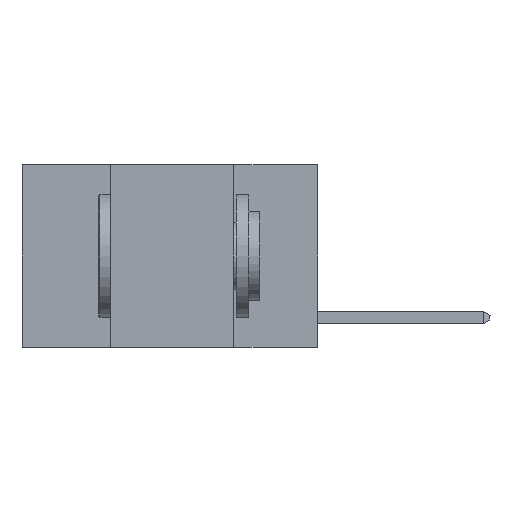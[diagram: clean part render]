
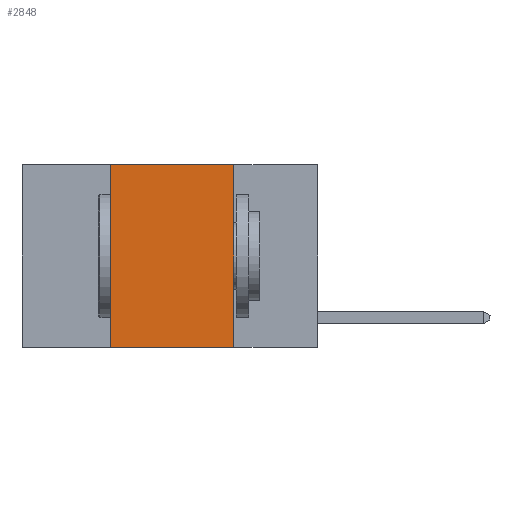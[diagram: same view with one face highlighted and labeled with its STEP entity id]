
A CAD part, left-side view. The second image highlights one B-rep face of the part: STEP entity #2848.
In plain terms, the highlighted planar face has unit normal (-1, 0, 0).
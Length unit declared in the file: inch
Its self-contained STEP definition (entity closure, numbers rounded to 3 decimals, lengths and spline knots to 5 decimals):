
#1011 = CARTESIAN_POINT ( 'NONE',  ( 0., 0.6, -0.37 ) ) ;
#1849 = ORIENTED_EDGE ( 'NONE', *, *, #4681, .T. ) ;
#1948 = LINE ( 'NONE', #10023, #14319 ) ;
#2730 = DIRECTION ( 'NONE',  ( 0., -1., 0. ) ) ;
#2848 = ADVANCED_FACE ( 'NONE', ( #12210 ), #6219, .F. ) ;
#2875 = ORIENTED_EDGE ( 'NONE', *, *, #22283, .F. ) ;
#3527 = CARTESIAN_POINT ( 'NONE',  ( 0., 0.42, -0.37 ) ) ;
#3731 = EDGE_CURVE ( 'NONE', #8537, #7631, #12191, .T. ) ;
#4681 = EDGE_CURVE ( 'NONE', #23251, #7631, #24128, .T. ) ;
#6219 = PLANE ( 'NONE',  #12428 ) ;
#6699 = CARTESIAN_POINT ( 'NONE',  ( 0., 0.6, 0. ) ) ;
#6808 = DIRECTION ( 'NONE',  ( 1., 0., 0. ) ) ;
#7631 = VERTEX_POINT ( 'NONE', #10575 ) ;
#7716 = VECTOR ( 'NONE', #7978, 39.37008 ) ;
#7978 = DIRECTION ( 'NONE',  ( 0., -1., 0. ) ) ;
#8537 = VERTEX_POINT ( 'NONE', #10747 ) ;
#8553 = DIRECTION ( 'NONE',  ( 0., 0., -1. ) ) ;
#10023 = CARTESIAN_POINT ( 'NONE',  ( 0., 0.42, 0. ) ) ;
#10090 = VERTEX_POINT ( 'NONE', #23191 ) ;
#10268 = DIRECTION ( 'NONE',  ( 0., 0., -1. ) ) ;
#10362 = VECTOR ( 'NONE', #10268, 39.37008 ) ;
#10408 = CARTESIAN_POINT ( 'NONE',  ( 0., 0.6, 0. ) ) ;
#10575 = CARTESIAN_POINT ( 'NONE',  ( 0., 0.17, -0.37 ) ) ;
#10747 = CARTESIAN_POINT ( 'NONE',  ( 0., 0.17, 0. ) ) ;
#12191 = LINE ( 'NONE', #23774, #10362 ) ;
#12210 = FACE_OUTER_BOUND ( 'NONE', #18554, .T. ) ;
#12391 = DIRECTION ( 'NONE',  ( 0., 0., 1. ) ) ;
#12428 = AXIS2_PLACEMENT_3D ( 'NONE', #10408, #6808, #8553 ) ;
#14319 = VECTOR ( 'NONE', #12391, 39.37008 ) ;
#16246 = ORIENTED_EDGE ( 'NONE', *, *, #16645, .F. ) ;
#16645 = EDGE_CURVE ( 'NONE', #10090, #8537, #18849, .T. ) ;
#18554 = EDGE_LOOP ( 'NONE', ( #19382, #16246, #2875, #1849 ) ) ;
#18849 = LINE ( 'NONE', #6699, #7716 ) ;
#19382 = ORIENTED_EDGE ( 'NONE', *, *, #3731, .F. ) ;
#21139 = VECTOR ( 'NONE', #2730, 39.37008 ) ;
#22283 = EDGE_CURVE ( 'NONE', #23251, #10090, #1948, .T. ) ;
#23191 = CARTESIAN_POINT ( 'NONE',  ( 0., 0.42, 0. ) ) ;
#23251 = VERTEX_POINT ( 'NONE', #3527 ) ;
#23774 = CARTESIAN_POINT ( 'NONE',  ( 0., 0.17, 0. ) ) ;
#24128 = LINE ( 'NONE', #1011, #21139 ) ;
